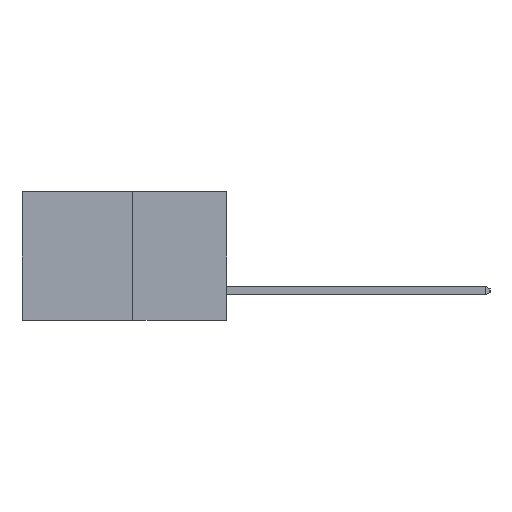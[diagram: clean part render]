
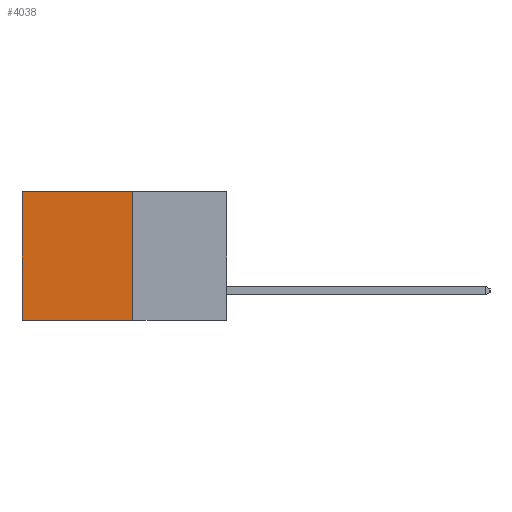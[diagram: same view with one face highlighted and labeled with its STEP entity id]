
A CAD part, left-side view. The second image highlights one B-rep face of the part: STEP entity #4038.
In plain terms, the highlighted planar face has unit normal (-1, 0, 0).
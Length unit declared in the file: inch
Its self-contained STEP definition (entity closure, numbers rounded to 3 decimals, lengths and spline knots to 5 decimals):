
#13 = LINE ( 'NONE', #8735, #4289 ) ;
#468 = EDGE_CURVE ( 'NONE', #3628, #2189, #13, .T. ) ;
#1448 = EDGE_LOOP ( 'NONE', ( #8546, #9572, #5571, #8196 ) ) ;
#1453 = DIRECTION ( 'NONE',  ( 1., 0., 0. ) ) ;
#1817 = CARTESIAN_POINT ( 'NONE',  ( 0.277, 0.59, -0.37 ) ) ;
#2007 = DIRECTION ( 'NONE',  ( 0., 0., -1. ) ) ;
#2189 = VERTEX_POINT ( 'NONE', #1817 ) ;
#2259 = CARTESIAN_POINT ( 'NONE',  ( 0.277, 0.59, -0.37 ) ) ;
#2619 = CARTESIAN_POINT ( 'NONE',  ( 0.277, 0.27, 0. ) ) ;
#3608 = DIRECTION ( 'NONE',  ( 0., 1., 0. ) ) ;
#3628 = VERTEX_POINT ( 'NONE', #5234 ) ;
#3748 = CARTESIAN_POINT ( 'NONE',  ( 0.277, 0.59, 0. ) ) ;
#3787 = VECTOR ( 'NONE', #2007, 39.37008 ) ;
#4038 = ADVANCED_FACE ( 'NONE', ( #9107 ), #8635, .F. ) ;
#4093 = VECTOR ( 'NONE', #7505, 39.37008 ) ;
#4289 = VECTOR ( 'NONE', #3608, 39.37008 ) ;
#4729 = VECTOR ( 'NONE', #9291, 39.37008 ) ;
#4807 = CARTESIAN_POINT ( 'NONE',  ( 0.277, 0.27, -0.37 ) ) ;
#5142 = CARTESIAN_POINT ( 'NONE',  ( 0.277, 0.27, 0. ) ) ;
#5234 = CARTESIAN_POINT ( 'NONE',  ( 0.277, 0.27, -0.37 ) ) ;
#5273 = CARTESIAN_POINT ( 'NONE',  ( 0.277, 0.27, -0.37 ) ) ;
#5439 = LINE ( 'NONE', #2259, #3787 ) ;
#5571 = ORIENTED_EDGE ( 'NONE', *, *, #9396, .F. ) ;
#5864 = EDGE_CURVE ( 'NONE', #10612, #2189, #5439, .T. ) ;
#6259 = LINE ( 'NONE', #2619, #4093 ) ;
#6713 = AXIS2_PLACEMENT_3D ( 'NONE', #4807, #1453, #9573 ) ;
#6871 = LINE ( 'NONE', #5273, #4729 ) ;
#7505 = DIRECTION ( 'NONE',  ( 0., 1., 0. ) ) ;
#8196 = ORIENTED_EDGE ( 'NONE', *, *, #8562, .T. ) ;
#8546 = ORIENTED_EDGE ( 'NONE', *, *, #5864, .T. ) ;
#8562 = EDGE_CURVE ( 'NONE', #9249, #10612, #6259, .T. ) ;
#8635 = PLANE ( 'NONE',  #6713 ) ;
#8735 = CARTESIAN_POINT ( 'NONE',  ( 0.277, 0.27, -0.37 ) ) ;
#9107 = FACE_OUTER_BOUND ( 'NONE', #1448, .T. ) ;
#9249 = VERTEX_POINT ( 'NONE', #5142 ) ;
#9291 = DIRECTION ( 'NONE',  ( 0., 0., -1. ) ) ;
#9396 = EDGE_CURVE ( 'NONE', #9249, #3628, #6871, .T. ) ;
#9572 = ORIENTED_EDGE ( 'NONE', *, *, #468, .F. ) ;
#9573 = DIRECTION ( 'NONE',  ( 0., 0., -1. ) ) ;
#10612 = VERTEX_POINT ( 'NONE', #3748 ) ;
